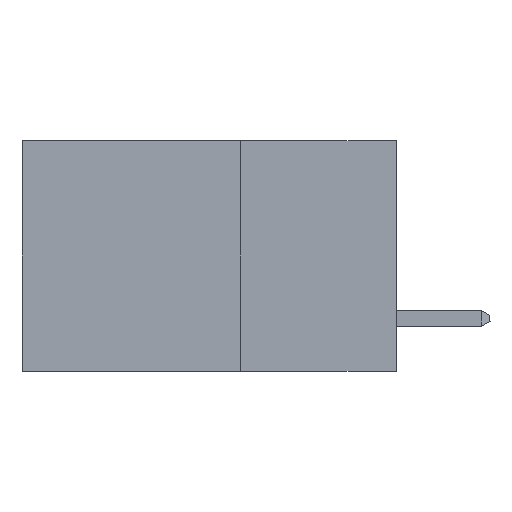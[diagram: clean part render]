
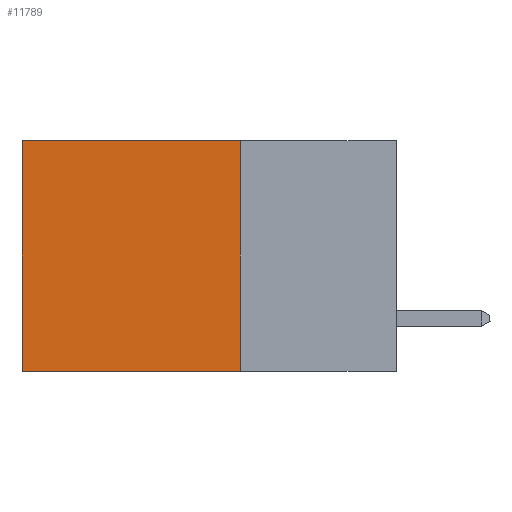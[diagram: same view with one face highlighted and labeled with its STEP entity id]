
A CAD part, left-side view. The second image highlights one B-rep face of the part: STEP entity #11789.
In plain terms, the highlighted planar face has unit normal (-1, 0, 0).
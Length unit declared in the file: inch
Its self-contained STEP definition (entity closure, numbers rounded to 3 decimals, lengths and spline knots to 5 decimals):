
#1149 = CARTESIAN_POINT ( 'NONE',  ( 0.298, 0.25, 0. ) ) ;
#1298 = LINE ( 'NONE', #15787, #17871 ) ;
#2551 = DIRECTION ( 'NONE',  ( 0., 0., -1. ) ) ;
#3219 = LINE ( 'NONE', #10748, #12790 ) ;
#3387 = CARTESIAN_POINT ( 'NONE',  ( 0.298, 0.6, -0.37 ) ) ;
#3421 = VECTOR ( 'NONE', #2551, 39.37008 ) ;
#4508 = AXIS2_PLACEMENT_3D ( 'NONE', #12922, #12785, #19287 ) ;
#5186 = CARTESIAN_POINT ( 'NONE',  ( 0.298, 0.6, 0. ) ) ;
#6594 = CARTESIAN_POINT ( 'NONE',  ( 0.298, 0.25, 0. ) ) ;
#7053 = CARTESIAN_POINT ( 'NONE',  ( 0.298, 0.6, 0. ) ) ;
#7693 = LINE ( 'NONE', #5186, #15756 ) ;
#7708 = EDGE_CURVE ( 'NONE', #17056, #8515, #3219, .T. ) ;
#7741 = CARTESIAN_POINT ( 'NONE',  ( 0.298, 0.25, -0.37 ) ) ;
#8232 = LINE ( 'NONE', #1149, #3421 ) ;
#8376 = ORIENTED_EDGE ( 'NONE', *, *, #7708, .T. ) ;
#8515 = VERTEX_POINT ( 'NONE', #7053 ) ;
#8945 = FACE_OUTER_BOUND ( 'NONE', #10222, .T. ) ;
#9161 = EDGE_CURVE ( 'NONE', #17056, #20689, #8232, .T. ) ;
#10060 = DIRECTION ( 'NONE',  ( 0., 0., -1. ) ) ;
#10222 = EDGE_LOOP ( 'NONE', ( #15168, #13308, #15761, #8376 ) ) ;
#10748 = CARTESIAN_POINT ( 'NONE',  ( 0.298, 0.25, 0. ) ) ;
#11789 = ADVANCED_FACE ( 'NONE', ( #8945 ), #17620, .F. ) ;
#12785 = DIRECTION ( 'NONE',  ( 1., 0., 0. ) ) ;
#12790 = VECTOR ( 'NONE', #20403, 39.37008 ) ;
#12922 = CARTESIAN_POINT ( 'NONE',  ( 0.298, 0.25, 0. ) ) ;
#13308 = ORIENTED_EDGE ( 'NONE', *, *, #14977, .F. ) ;
#14977 = EDGE_CURVE ( 'NONE', #20689, #20328, #1298, .T. ) ;
#15168 = ORIENTED_EDGE ( 'NONE', *, *, #19772, .T. ) ;
#15756 = VECTOR ( 'NONE', #10060, 39.37008 ) ;
#15761 = ORIENTED_EDGE ( 'NONE', *, *, #9161, .F. ) ;
#15787 = CARTESIAN_POINT ( 'NONE',  ( 0.298, 0.25, -0.37 ) ) ;
#17056 = VERTEX_POINT ( 'NONE', #6594 ) ;
#17620 = PLANE ( 'NONE',  #4508 ) ;
#17871 = VECTOR ( 'NONE', #20474, 39.37008 ) ;
#19287 = DIRECTION ( 'NONE',  ( 0., 0., -1. ) ) ;
#19772 = EDGE_CURVE ( 'NONE', #8515, #20328, #7693, .T. ) ;
#20328 = VERTEX_POINT ( 'NONE', #3387 ) ;
#20403 = DIRECTION ( 'NONE',  ( 0., 1., 0. ) ) ;
#20474 = DIRECTION ( 'NONE',  ( 0., 1., 0. ) ) ;
#20689 = VERTEX_POINT ( 'NONE', #7741 ) ;
